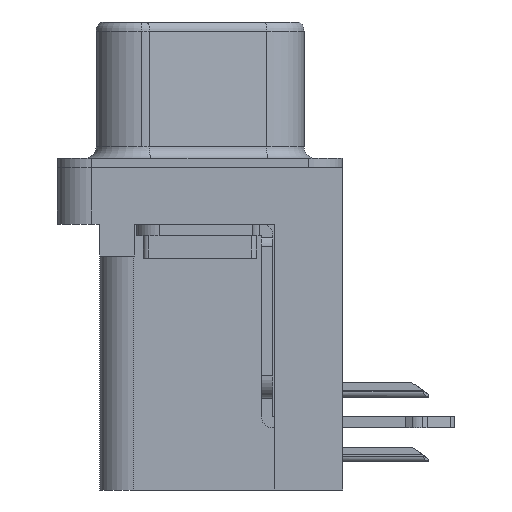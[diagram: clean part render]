
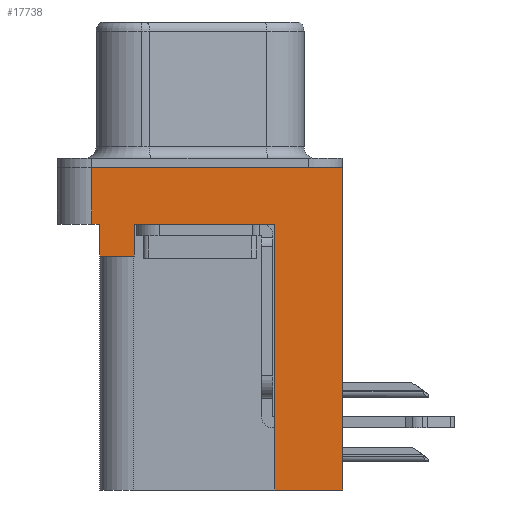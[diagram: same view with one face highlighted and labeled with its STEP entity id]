
A CAD part, left-side view. The second image highlights one B-rep face of the part: STEP entity #17738.
In plain terms, the highlighted planar face has unit normal (-1, 0, 0).
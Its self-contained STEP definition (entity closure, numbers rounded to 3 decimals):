
#133 = LINE ( 'NONE', #7929, #6430 ) ;
#282 = DIRECTION ( 'NONE',  ( 0., -1., 0. ) ) ;
#319 = DIRECTION ( 'NONE',  ( 0., 0., 1. ) ) ;
#399 = VECTOR ( 'NONE', #5503, 1000. ) ;
#440 = VERTEX_POINT ( 'NONE', #4980 ) ;
#634 = VECTOR ( 'NONE', #282, 1000. ) ;
#820 = CARTESIAN_POINT ( 'NONE',  ( -2.91, -6.275, -2.5 ) ) ;
#1140 = VERTEX_POINT ( 'NONE', #21674 ) ;
#1585 = CARTESIAN_POINT ( 'NONE',  ( -2.91, -3.295, -14.2 ) ) ;
#1778 = CARTESIAN_POINT ( 'NONE',  ( -2.91, 2.895, -2.5 ) ) ;
#1833 = CARTESIAN_POINT ( 'NONE',  ( -2.91, 4.425, -3.9 ) ) ;
#2431 = DIRECTION ( 'NONE',  ( 0., 0., 1. ) ) ;
#2557 = ORIENTED_EDGE ( 'NONE', *, *, #2804, .T. ) ;
#2804 = EDGE_CURVE ( 'NONE', #3079, #23627, #11090, .T. ) ;
#3079 = VERTEX_POINT ( 'NONE', #1778 ) ;
#3315 = ORIENTED_EDGE ( 'NONE', *, *, #9744, .F. ) ;
#3339 = CARTESIAN_POINT ( 'NONE',  ( -2.91, -3.295, -14.2 ) ) ;
#3698 = DIRECTION ( 'NONE',  ( 0., 1., 0. ) ) ;
#3941 = CARTESIAN_POINT ( 'NONE',  ( -2.91, -6.275, -2.5 ) ) ;
#4227 = EDGE_CURVE ( 'NONE', #16320, #21885, #8578, .T. ) ;
#4313 = AXIS2_PLACEMENT_3D ( 'NONE', #22630, #24427, #11075 ) ;
#4374 = EDGE_LOOP ( 'NONE', ( #17519, #18084, #8738, #3315, #22707, #11271, #2557, #14941, #19928, #25028 ) ) ;
#4980 = CARTESIAN_POINT ( 'NONE',  ( -2.91, -6.275, -14.2 ) ) ;
#5093 = CARTESIAN_POINT ( 'NONE',  ( -2.91, -3.295, -2.5 ) ) ;
#5384 = CARTESIAN_POINT ( 'NONE',  ( -2.91, 4.775, 0. ) ) ;
#5503 = DIRECTION ( 'NONE',  ( 0., 1., 0. ) ) ;
#5562 = LINE ( 'NONE', #1585, #17493 ) ;
#5623 = CARTESIAN_POINT ( 'NONE',  ( -2.91, 4.425, -3.9 ) ) ;
#5727 = LINE ( 'NONE', #13607, #9334 ) ;
#6118 = LINE ( 'NONE', #3941, #18102 ) ;
#6291 = EDGE_CURVE ( 'NONE', #1140, #16320, #5727, .T. ) ;
#6430 = VECTOR ( 'NONE', #2431, 1000. ) ;
#6919 = VECTOR ( 'NONE', #3698, 1000. ) ;
#6935 = EDGE_CURVE ( 'NONE', #440, #11838, #11225, .T. ) ;
#7657 = LINE ( 'NONE', #5623, #6919 ) ;
#7929 = CARTESIAN_POINT ( 'NONE',  ( -2.91, 2.895, -3.9 ) ) ;
#8578 = LINE ( 'NONE', #21898, #634 ) ;
#8738 = ORIENTED_EDGE ( 'NONE', *, *, #17803, .T. ) ;
#8925 = FACE_OUTER_BOUND ( 'NONE', #4374, .T. ) ;
#9334 = VECTOR ( 'NONE', #22999, 1000. ) ;
#9411 = CARTESIAN_POINT ( 'NONE',  ( -2.91, 4.425, -2.5 ) ) ;
#9744 = EDGE_CURVE ( 'NONE', #20083, #9754, #22744, .T. ) ;
#9754 = VERTEX_POINT ( 'NONE', #9411 ) ;
#10600 = CARTESIAN_POINT ( 'NONE',  ( -2.91, -6.275, -2.5 ) ) ;
#11075 = DIRECTION ( 'NONE',  ( 0., 0., 1. ) ) ;
#11090 = LINE ( 'NONE', #10600, #23453 ) ;
#11225 = LINE ( 'NONE', #3339, #399 ) ;
#11271 = ORIENTED_EDGE ( 'NONE', *, *, #16388, .T. ) ;
#11838 = VERTEX_POINT ( 'NONE', #14461 ) ;
#13217 = DIRECTION ( 'NONE',  ( 0., 0., 1. ) ) ;
#13607 = CARTESIAN_POINT ( 'NONE',  ( -2.91, 4.775, -2.5 ) ) ;
#13872 = DIRECTION ( 'NONE',  ( 0., -1., 0. ) ) ;
#14461 = CARTESIAN_POINT ( 'NONE',  ( -2.91, -3.295, -14.2 ) ) ;
#14897 = CARTESIAN_POINT ( 'NONE',  ( -2.91, 4.425, -3.9 ) ) ;
#14941 = ORIENTED_EDGE ( 'NONE', *, *, #25006, .F. ) ;
#15158 = CARTESIAN_POINT ( 'NONE',  ( -2.91, -6.275, 0. ) ) ;
#16030 = VERTEX_POINT ( 'NONE', #22975 ) ;
#16320 = VERTEX_POINT ( 'NONE', #5384 ) ;
#16388 = EDGE_CURVE ( 'NONE', #16030, #3079, #133, .T. ) ;
#16666 = PLANE ( 'NONE',  #4313 ) ;
#17493 = VECTOR ( 'NONE', #20550, 1000. ) ;
#17519 = ORIENTED_EDGE ( 'NONE', *, *, #4227, .F. ) ;
#17738 = ADVANCED_FACE ( 'NONE', ( #8925 ), #16666, .T. ) ;
#17803 = EDGE_CURVE ( 'NONE', #1140, #9754, #6118, .T. ) ;
#17907 = VECTOR ( 'NONE', #319, 1000. ) ;
#18084 = ORIENTED_EDGE ( 'NONE', *, *, #6291, .F. ) ;
#18102 = VECTOR ( 'NONE', #13872, 1000. ) ;
#19540 = VECTOR ( 'NONE', #13217, 1000. ) ;
#19928 = ORIENTED_EDGE ( 'NONE', *, *, #6935, .F. ) ;
#20083 = VERTEX_POINT ( 'NONE', #1833 ) ;
#20550 = DIRECTION ( 'NONE',  ( 0., 0., 1. ) ) ;
#21565 = LINE ( 'NONE', #820, #17907 ) ;
#21674 = CARTESIAN_POINT ( 'NONE',  ( -2.91, 4.775, -2.5 ) ) ;
#21885 = VERTEX_POINT ( 'NONE', #15158 ) ;
#21898 = CARTESIAN_POINT ( 'NONE',  ( -2.91, -6.275, 0. ) ) ;
#21959 = EDGE_CURVE ( 'NONE', #16030, #20083, #7657, .T. ) ;
#22630 = CARTESIAN_POINT ( 'NONE',  ( -2.91, -6.275, -2.5 ) ) ;
#22707 = ORIENTED_EDGE ( 'NONE', *, *, #21959, .F. ) ;
#22744 = LINE ( 'NONE', #14897, #19540 ) ;
#22958 = EDGE_CURVE ( 'NONE', #440, #21885, #21565, .T. ) ;
#22975 = CARTESIAN_POINT ( 'NONE',  ( -2.91, 2.895, -3.9 ) ) ;
#22999 = DIRECTION ( 'NONE',  ( 0., 0., 1. ) ) ;
#23453 = VECTOR ( 'NONE', #24075, 1000. ) ;
#23627 = VERTEX_POINT ( 'NONE', #5093 ) ;
#24075 = DIRECTION ( 'NONE',  ( 0., -1., 0. ) ) ;
#24427 = DIRECTION ( 'NONE',  ( -1., 0., 0. ) ) ;
#25006 = EDGE_CURVE ( 'NONE', #11838, #23627, #5562, .T. ) ;
#25028 = ORIENTED_EDGE ( 'NONE', *, *, #22958, .T. ) ;
